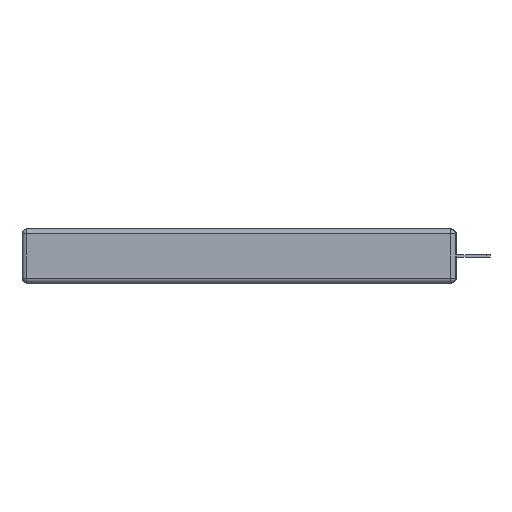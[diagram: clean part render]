
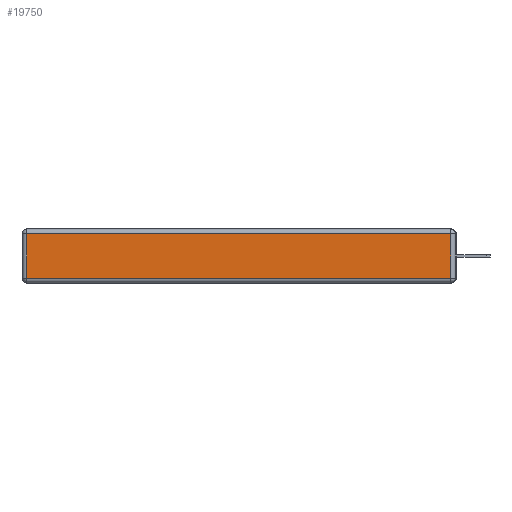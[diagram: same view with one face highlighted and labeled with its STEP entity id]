
A CAD part, left-side view. The second image highlights one B-rep face of the part: STEP entity #19750.
In plain terms, the highlighted planar face has unit normal (-1, 0, 0).
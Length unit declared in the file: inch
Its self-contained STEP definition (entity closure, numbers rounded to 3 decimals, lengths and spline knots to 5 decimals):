
#414 = VERTEX_POINT ( 'NONE', #9513 ) ;
#518 = EDGE_LOOP ( 'NONE', ( #9327, #3861, #16699, #7416 ) ) ;
#3301 = CARTESIAN_POINT ( 'NONE',  ( 0., 0., -0.313 ) ) ;
#3334 = EDGE_CURVE ( 'NONE', #9059, #414, #19449, .T. ) ;
#3861 = ORIENTED_EDGE ( 'NONE', *, *, #3334, .T. ) ;
#4242 = DIRECTION ( 'NONE',  ( 0., 0., -1. ) ) ;
#4579 = DIRECTION ( 'NONE',  ( -1., 0., 0. ) ) ;
#4881 = DIRECTION ( 'NONE',  ( 0., -1., 0. ) ) ;
#7056 = VECTOR ( 'NONE', #4242, 39.37008 ) ;
#7416 = ORIENTED_EDGE ( 'NONE', *, *, #18059, .T. ) ;
#7448 = CARTESIAN_POINT ( 'NONE',  ( 0., 2.72, -0.343 ) ) ;
#7756 = DIRECTION ( 'NONE',  ( 0., 0., 1. ) ) ;
#8148 = VECTOR ( 'NONE', #16449, 39.37008 ) ;
#9059 = VERTEX_POINT ( 'NONE', #18183 ) ;
#9145 = CARTESIAN_POINT ( 'NONE',  ( 0., 2.72, -0.313 ) ) ;
#9209 = LINE ( 'NONE', #3301, #16971 ) ;
#9327 = ORIENTED_EDGE ( 'NONE', *, *, #16864, .T. ) ;
#9513 = CARTESIAN_POINT ( 'NONE',  ( 0., 0.03, -0.03 ) ) ;
#10264 = EDGE_CURVE ( 'NONE', #414, #20167, #15938, .T. ) ;
#10286 = CARTESIAN_POINT ( 'NONE',  ( 0., 2.75, -0.03 ) ) ;
#13535 = VERTEX_POINT ( 'NONE', #9145 ) ;
#13980 = PLANE ( 'NONE',  #16614 ) ;
#15223 = CARTESIAN_POINT ( 'NONE',  ( 0., 2.72, -0.03 ) ) ;
#15396 = VECTOR ( 'NONE', #7756, 39.37008 ) ;
#15584 = DIRECTION ( 'NONE',  ( 0., 0., 1. ) ) ;
#15784 = FACE_OUTER_BOUND ( 'NONE', #518, .T. ) ;
#15857 = LINE ( 'NONE', #7448, #7056 ) ;
#15938 = LINE ( 'NONE', #10286, #8148 ) ;
#16449 = DIRECTION ( 'NONE',  ( 0., 1., 0. ) ) ;
#16614 = AXIS2_PLACEMENT_3D ( 'NONE', #17057, #4579, #15584 ) ;
#16699 = ORIENTED_EDGE ( 'NONE', *, *, #10264, .T. ) ;
#16864 = EDGE_CURVE ( 'NONE', #13535, #9059, #9209, .T. ) ;
#16971 = VECTOR ( 'NONE', #4881, 39.37008 ) ;
#17057 = CARTESIAN_POINT ( 'NONE',  ( 0., 0., -0.343 ) ) ;
#18059 = EDGE_CURVE ( 'NONE', #20167, #13535, #15857, .T. ) ;
#18183 = CARTESIAN_POINT ( 'NONE',  ( 0., 0.03, -0.313 ) ) ;
#19208 = CARTESIAN_POINT ( 'NONE',  ( 0., 0.03, -0.343 ) ) ;
#19449 = LINE ( 'NONE', #19208, #15396 ) ;
#19750 = ADVANCED_FACE ( 'NONE', ( #15784 ), #13980, .T. ) ;
#20167 = VERTEX_POINT ( 'NONE', #15223 ) ;
